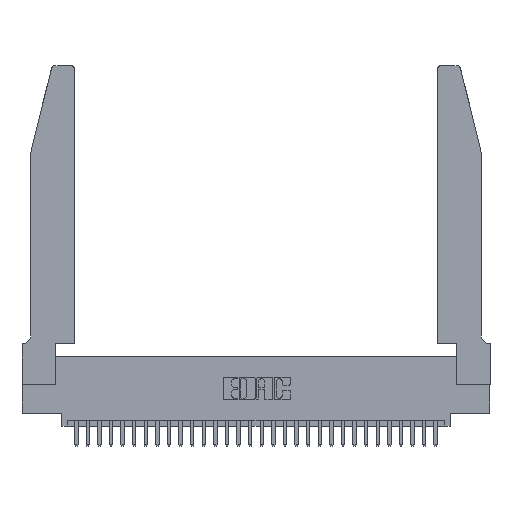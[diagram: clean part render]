
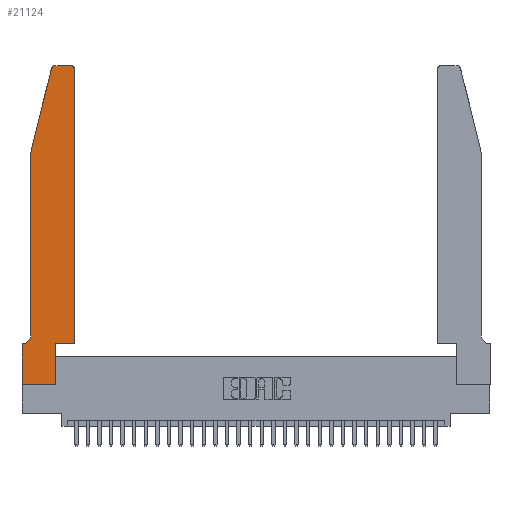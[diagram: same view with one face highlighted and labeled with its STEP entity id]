
A CAD part, top view. The second image highlights one B-rep face of the part: STEP entity #21124.
In plain terms, the highlighted planar face has unit normal (0, 0, 1).
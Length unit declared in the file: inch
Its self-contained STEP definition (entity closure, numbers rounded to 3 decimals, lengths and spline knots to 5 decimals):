
#6 = CARTESIAN_POINT ( 'NONE',  ( 0.284, 2.75, 0.37 ) ) ;
#95 = VECTOR ( 'NONE', #24347, 39.37008 ) ;
#121 = CARTESIAN_POINT ( 'NONE',  ( 0.0055, 0.35, 0.37 ) ) ;
#406 = CARTESIAN_POINT ( 'NONE',  ( 0.2605, 2.75, 0.37 ) ) ;
#613 = VECTOR ( 'NONE', #14939, 39.37008 ) ;
#753 = VERTEX_POINT ( 'NONE', #13840 ) ;
#780 = VERTEX_POINT ( 'NONE', #1451 ) ;
#791 = CARTESIAN_POINT ( 'NONE',  ( 0.2865, 0., 0.37 ) ) ;
#975 = DIRECTION ( 'NONE',  ( 1., 0., 0. ) ) ;
#1145 = VECTOR ( 'NONE', #28855, 39.37008 ) ;
#1371 = DIRECTION ( 'NONE',  ( 0., 0., -1. ) ) ;
#1451 = CARTESIAN_POINT ( 'NONE',  ( 0.0755, 0.42, 0.37 ) ) ;
#2702 = DIRECTION ( 'NONE',  ( 1., 0., 0. ) ) ;
#3402 = VECTOR ( 'NONE', #2702, 39.37008 ) ;
#3466 = VERTEX_POINT ( 'NONE', #18914 ) ;
#3662 = ORIENTED_EDGE ( 'NONE', *, *, #24081, .T. ) ;
#3681 = DIRECTION ( 'NONE',  ( 0., -1., 0. ) ) ;
#3687 = VECTOR ( 'NONE', #3681, 39.37008 ) ;
#3719 = EDGE_CURVE ( 'NONE', #780, #17936, #29353, .T. ) ;
#3825 = LINE ( 'NONE', #28659, #1145 ) ;
#4266 = CIRCLE ( 'NONE', #5270, 0.03 ) ;
#4519 = EDGE_CURVE ( 'NONE', #7998, #29332, #30910, .T. ) ;
#4549 = CARTESIAN_POINT ( 'NONE',  ( 0.4505, 0.35, 0.37 ) ) ;
#4564 = EDGE_CURVE ( 'NONE', #753, #17898, #13091, .T. ) ;
#4979 = VERTEX_POINT ( 'NONE', #791 ) ;
#5270 = AXIS2_PLACEMENT_3D ( 'NONE', #5936, #22890, #975 ) ;
#5332 = EDGE_CURVE ( 'NONE', #17898, #7998, #4266, .T. ) ;
#5674 = AXIS2_PLACEMENT_3D ( 'NONE', #13184, #25458, #27790 ) ;
#5826 = ORIENTED_EDGE ( 'NONE', *, *, #24561, .T. ) ;
#5936 = CARTESIAN_POINT ( 'NONE',  ( 0.284, 2.72, 0.37 ) ) ;
#6499 = CARTESIAN_POINT ( 'NONE',  ( 0.2865, 0.35, 0.37 ) ) ;
#6761 = DIRECTION ( 'NONE',  ( 0., 1., 0. ) ) ;
#7998 = VERTEX_POINT ( 'NONE', #28839 ) ;
#8219 = FACE_OUTER_BOUND ( 'NONE', #9113, .T. ) ;
#8652 = LINE ( 'NONE', #21260, #17727 ) ;
#9113 = EDGE_LOOP ( 'NONE', ( #19742, #17415, #23308, #10511, #19878, #3662, #5826, #22993, #20665, #18134, #14081, #13249 ) ) ;
#9951 = CARTESIAN_POINT ( 'NONE',  ( 0.0755, 2., 0.37 ) ) ;
#10050 = EDGE_CURVE ( 'NONE', #4979, #18822, #27169, .T. ) ;
#10061 = DIRECTION ( 'NONE',  ( -0.239, -0.971, 0. ) ) ;
#10511 = ORIENTED_EDGE ( 'NONE', *, *, #31171, .T. ) ;
#11022 = LINE ( 'NONE', #4549, #20045 ) ;
#11030 = CARTESIAN_POINT ( 'NONE',  ( 0.4205, 2.72, 0.37 ) ) ;
#11458 = CARTESIAN_POINT ( 'NONE',  ( 0.0755, 2., 0.37 ) ) ;
#13091 = LINE ( 'NONE', #406, #95 ) ;
#13184 = CARTESIAN_POINT ( 'NONE',  ( 0., 0.35, 0.37 ) ) ;
#13249 = ORIENTED_EDGE ( 'NONE', *, *, #14442, .T. ) ;
#13571 = DIRECTION ( 'NONE',  ( 1., 0., 0. ) ) ;
#13840 = CARTESIAN_POINT ( 'NONE',  ( 0.4205, 2.75, 0.37 ) ) ;
#13862 = VECTOR ( 'NONE', #10061, 39.37008 ) ;
#14081 = ORIENTED_EDGE ( 'NONE', *, *, #25378, .T. ) ;
#14317 = AXIS2_PLACEMENT_3D ( 'NONE', #11030, #27954, #13571 ) ;
#14442 = EDGE_CURVE ( 'NONE', #20210, #753, #21536, .T. ) ;
#14939 = DIRECTION ( 'NONE',  ( 0., -1., 0. ) ) ;
#15802 = VECTOR ( 'NONE', #23663, 39.37008 ) ;
#15905 = CARTESIAN_POINT ( 'NONE',  ( 0., 0., 0.37 ) ) ;
#17415 = ORIENTED_EDGE ( 'NONE', *, *, #5332, .T. ) ;
#17727 = VECTOR ( 'NONE', #6761, 39.37008 ) ;
#17898 = VERTEX_POINT ( 'NONE', #6 ) ;
#17936 = VERTEX_POINT ( 'NONE', #121 ) ;
#18134 = ORIENTED_EDGE ( 'NONE', *, *, #19145, .T. ) ;
#18168 = LINE ( 'NONE', #11458, #613 ) ;
#18636 = CARTESIAN_POINT ( 'NONE',  ( 0.4505, 2.72, 0.37 ) ) ;
#18822 = VERTEX_POINT ( 'NONE', #25591 ) ;
#18914 = CARTESIAN_POINT ( 'NONE',  ( 0., 0.35, 0.37 ) ) ;
#19145 = EDGE_CURVE ( 'NONE', #18822, #28275, #11022, .T. ) ;
#19742 = ORIENTED_EDGE ( 'NONE', *, *, #4564, .T. ) ;
#19878 = ORIENTED_EDGE ( 'NONE', *, *, #3719, .T. ) ;
#20045 = VECTOR ( 'NONE', #24705, 39.37008 ) ;
#20132 = PLANE ( 'NONE',  #5674 ) ;
#20210 = VERTEX_POINT ( 'NONE', #18636 ) ;
#20665 = ORIENTED_EDGE ( 'NONE', *, *, #10050, .T. ) ;
#20693 = AXIS2_PLACEMENT_3D ( 'NONE', #22984, #1371, #30272 ) ;
#21124 = ADVANCED_FACE ( 'NONE', ( #8219 ), #20132, .T. ) ;
#21260 = CARTESIAN_POINT ( 'NONE',  ( 0.4505, 0.35, 0.37 ) ) ;
#21536 = CIRCLE ( 'NONE', #14317, 0.03 ) ;
#22890 = DIRECTION ( 'NONE',  ( 0., 0., 1. ) ) ;
#22984 = CARTESIAN_POINT ( 'NONE',  ( 0.0055, 0.42, 0.37 ) ) ;
#22993 = ORIENTED_EDGE ( 'NONE', *, *, #29342, .T. ) ;
#23087 = LINE ( 'NONE', #15905, #3687 ) ;
#23308 = ORIENTED_EDGE ( 'NONE', *, *, #4519, .T. ) ;
#23663 = DIRECTION ( 'NONE',  ( 0., 1., 0. ) ) ;
#24081 = EDGE_CURVE ( 'NONE', #17936, #3466, #3825, .T. ) ;
#24347 = DIRECTION ( 'NONE',  ( -1., 0., 0. ) ) ;
#24561 = EDGE_CURVE ( 'NONE', #3466, #30620, #23087, .T. ) ;
#24705 = DIRECTION ( 'NONE',  ( 1., 0., 0. ) ) ;
#24783 = CARTESIAN_POINT ( 'NONE',  ( 0.4505, 0.35, 0.37 ) ) ;
#25378 = EDGE_CURVE ( 'NONE', #28275, #20210, #8652, .T. ) ;
#25458 = DIRECTION ( 'NONE',  ( 0., 0., 1. ) ) ;
#25591 = CARTESIAN_POINT ( 'NONE',  ( 0.2865, 0.35, 0.37 ) ) ;
#27169 = LINE ( 'NONE', #6499, #15802 ) ;
#27727 = LINE ( 'NONE', #29379, #3402 ) ;
#27790 = DIRECTION ( 'NONE',  ( 1., 0., 0. ) ) ;
#27954 = DIRECTION ( 'NONE',  ( 0., 0., 1. ) ) ;
#28275 = VERTEX_POINT ( 'NONE', #24783 ) ;
#28659 = CARTESIAN_POINT ( 'NONE',  ( 0.0755, 0.35, 0.37 ) ) ;
#28839 = CARTESIAN_POINT ( 'NONE',  ( 0.25487, 2.72718, 0.37 ) ) ;
#28855 = DIRECTION ( 'NONE',  ( -1., 0., 0. ) ) ;
#29267 = CARTESIAN_POINT ( 'NONE',  ( 0.0755, 2., 0.37 ) ) ;
#29332 = VERTEX_POINT ( 'NONE', #29267 ) ;
#29342 = EDGE_CURVE ( 'NONE', #30620, #4979, #27727, .T. ) ;
#29353 = CIRCLE ( 'NONE', #20693, 0.07 ) ;
#29379 = CARTESIAN_POINT ( 'NONE',  ( 0., 0., 0.37 ) ) ;
#30272 = DIRECTION ( 'NONE',  ( -1., 0., 0. ) ) ;
#30620 = VERTEX_POINT ( 'NONE', #31284 ) ;
#30910 = LINE ( 'NONE', #9951, #13862 ) ;
#31171 = EDGE_CURVE ( 'NONE', #29332, #780, #18168, .T. ) ;
#31284 = CARTESIAN_POINT ( 'NONE',  ( 0., 0., 0.37 ) ) ;
